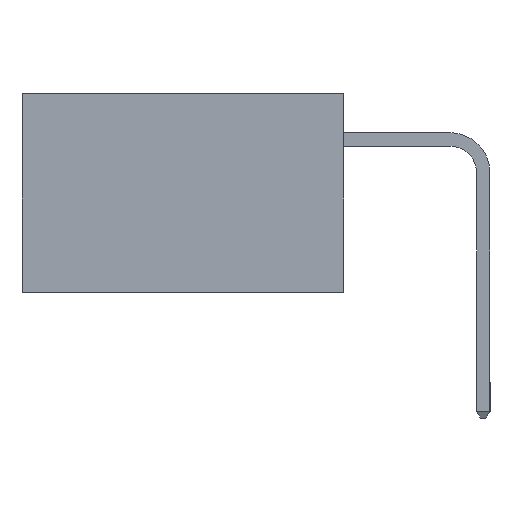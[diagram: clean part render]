
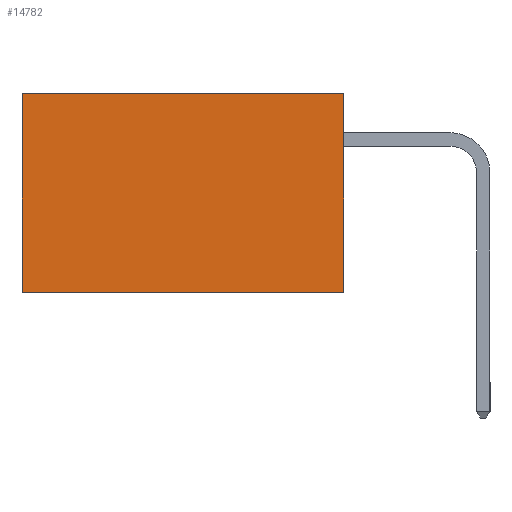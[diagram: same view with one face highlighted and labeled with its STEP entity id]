
A CAD part, left-side view. The second image highlights one B-rep face of the part: STEP entity #14782.
In plain terms, the highlighted planar face has unit normal (-1, 0, 0).
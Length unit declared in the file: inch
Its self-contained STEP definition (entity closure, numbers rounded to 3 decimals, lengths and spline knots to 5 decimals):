
#53 = DIRECTION ( 'NONE',  ( 0., 1., 0. ) ) ;
#173 = FACE_OUTER_BOUND ( 'NONE', #11535, .T. ) ;
#1217 = VECTOR ( 'NONE', #5004, 39.37008 ) ;
#1418 = CARTESIAN_POINT ( 'NONE',  ( 0.298, 0.6, 0. ) ) ;
#1637 = VECTOR ( 'NONE', #53, 39.37008 ) ;
#2763 = DIRECTION ( 'NONE',  ( 0., 0., -1. ) ) ;
#3667 = VECTOR ( 'NONE', #2763, 39.37008 ) ;
#5004 = DIRECTION ( 'NONE',  ( 0., 1., 0. ) ) ;
#5212 = LINE ( 'NONE', #14466, #1637 ) ;
#5516 = PLANE ( 'NONE',  #14475 ) ;
#5538 = VERTEX_POINT ( 'NONE', #5678 ) ;
#5678 = CARTESIAN_POINT ( 'NONE',  ( 0.298, 0.6, 0. ) ) ;
#5707 = ORIENTED_EDGE ( 'NONE', *, *, #16647, .T. ) ;
#5755 = CARTESIAN_POINT ( 'NONE',  ( 0.298, 0., 0. ) ) ;
#5769 = ORIENTED_EDGE ( 'NONE', *, *, #14512, .T. ) ;
#6453 = ORIENTED_EDGE ( 'NONE', *, *, #10030, .F. ) ;
#6832 = DIRECTION ( 'NONE',  ( 1., 0., 0. ) ) ;
#8254 = EDGE_CURVE ( 'NONE', #14200, #14061, #12966, .T. ) ;
#8389 = ORIENTED_EDGE ( 'NONE', *, *, #8254, .F. ) ;
#9609 = VECTOR ( 'NONE', #11242, 39.37008 ) ;
#10030 = EDGE_CURVE ( 'NONE', #14061, #10205, #5212, .T. ) ;
#10205 = VERTEX_POINT ( 'NONE', #13592 ) ;
#10667 = LINE ( 'NONE', #1418, #3667 ) ;
#11242 = DIRECTION ( 'NONE',  ( 0., 0., -1. ) ) ;
#11535 = EDGE_LOOP ( 'NONE', ( #5707, #6453, #8389, #5769 ) ) ;
#11742 = LINE ( 'NONE', #14071, #1217 ) ;
#12966 = LINE ( 'NONE', #13249, #9609 ) ;
#13232 = CARTESIAN_POINT ( 'NONE',  ( 0.298, 0., -0.37 ) ) ;
#13249 = CARTESIAN_POINT ( 'NONE',  ( 0.298, 0., 0. ) ) ;
#13268 = CARTESIAN_POINT ( 'NONE',  ( 0.298, 0., 0. ) ) ;
#13592 = CARTESIAN_POINT ( 'NONE',  ( 0.298, 0.6, -0.37 ) ) ;
#14061 = VERTEX_POINT ( 'NONE', #13232 ) ;
#14071 = CARTESIAN_POINT ( 'NONE',  ( 0.298, 0., 0. ) ) ;
#14200 = VERTEX_POINT ( 'NONE', #5755 ) ;
#14466 = CARTESIAN_POINT ( 'NONE',  ( 0.298, 0., -0.37 ) ) ;
#14475 = AXIS2_PLACEMENT_3D ( 'NONE', #13268, #6832, #15897 ) ;
#14512 = EDGE_CURVE ( 'NONE', #14200, #5538, #11742, .T. ) ;
#14782 = ADVANCED_FACE ( 'NONE', ( #173 ), #5516, .F. ) ;
#15897 = DIRECTION ( 'NONE',  ( 0., 0., -1. ) ) ;
#16647 = EDGE_CURVE ( 'NONE', #5538, #10205, #10667, .T. ) ;
